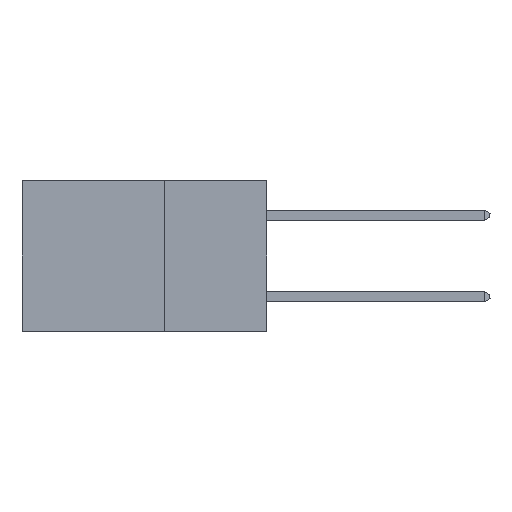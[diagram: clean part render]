
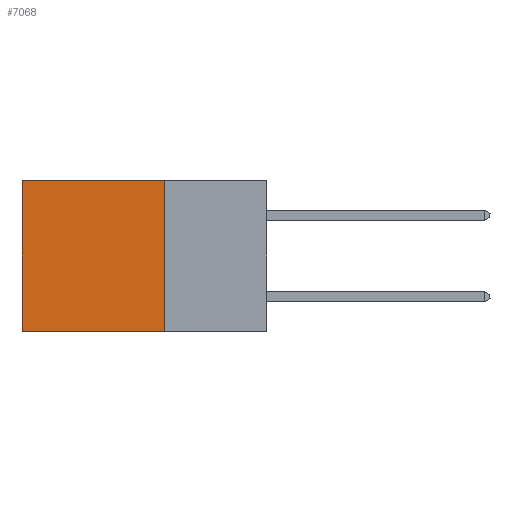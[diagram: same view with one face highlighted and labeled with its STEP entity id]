
A CAD part, left-side view. The second image highlights one B-rep face of the part: STEP entity #7068.
In plain terms, the highlighted planar face has unit normal (-1, 0, 0).
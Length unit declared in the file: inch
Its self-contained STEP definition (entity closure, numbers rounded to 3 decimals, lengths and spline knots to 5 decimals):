
#1151 = CARTESIAN_POINT ( 'NONE',  ( 0.2875, 0.25, 0. ) ) ;
#1280 = CARTESIAN_POINT ( 'NONE',  ( 0.2875, 0.25, -0.37 ) ) ;
#2963 = DIRECTION ( 'NONE',  ( 0., 0., -1. ) ) ;
#4629 = DIRECTION ( 'NONE',  ( 1., 0., 0. ) ) ;
#5916 = CARTESIAN_POINT ( 'NONE',  ( 0.2875, 0.25, 0. ) ) ;
#7068 = ADVANCED_FACE ( 'NONE', ( #40248 ), #21958, .F. ) ;
#8092 = EDGE_CURVE ( 'NONE', #14095, #40239, #42843, .T. ) ;
#14095 = VERTEX_POINT ( 'NONE', #38770 ) ;
#14405 = VERTEX_POINT ( 'NONE', #30082 ) ;
#14939 = ORIENTED_EDGE ( 'NONE', *, *, #38600, .T. ) ;
#16433 = DIRECTION ( 'NONE',  ( 0., 0., -1. ) ) ;
#17549 = LINE ( 'NONE', #37400, #34756 ) ;
#18613 = DIRECTION ( 'NONE',  ( 0., 1., 0. ) ) ;
#20931 = EDGE_CURVE ( 'NONE', #40239, #34434, #23187, .T. ) ;
#21083 = CARTESIAN_POINT ( 'NONE',  ( 0.2875, 0.6, -0.37 ) ) ;
#21958 = PLANE ( 'NONE',  #38261 ) ;
#23187 = LINE ( 'NONE', #1280, #41395 ) ;
#25270 = VECTOR ( 'NONE', #30795, 39.37008 ) ;
#27459 = EDGE_LOOP ( 'NONE', ( #14939, #30585, #40939, #38949 ) ) ;
#28905 = DIRECTION ( 'NONE',  ( 0., 0., -1. ) ) ;
#30082 = CARTESIAN_POINT ( 'NONE',  ( 0.2875, 0.6, 0. ) ) ;
#30585 = ORIENTED_EDGE ( 'NONE', *, *, #20931, .F. ) ;
#30795 = DIRECTION ( 'NONE',  ( 0., 1., 0. ) ) ;
#32689 = VECTOR ( 'NONE', #16433, 39.37008 ) ;
#32819 = CARTESIAN_POINT ( 'NONE',  ( 0.2875, 0.25, -0.37 ) ) ;
#34368 = LINE ( 'NONE', #40932, #25270 ) ;
#34434 = VERTEX_POINT ( 'NONE', #21083 ) ;
#34756 = VECTOR ( 'NONE', #2963, 39.37008 ) ;
#37015 = EDGE_CURVE ( 'NONE', #14095, #14405, #34368, .T. ) ;
#37400 = CARTESIAN_POINT ( 'NONE',  ( 0.2875, 0.6, 0. ) ) ;
#38261 = AXIS2_PLACEMENT_3D ( 'NONE', #1151, #4629, #28905 ) ;
#38600 = EDGE_CURVE ( 'NONE', #14405, #34434, #17549, .T. ) ;
#38770 = CARTESIAN_POINT ( 'NONE',  ( 0.2875, 0.25, 0. ) ) ;
#38949 = ORIENTED_EDGE ( 'NONE', *, *, #37015, .T. ) ;
#40239 = VERTEX_POINT ( 'NONE', #32819 ) ;
#40248 = FACE_OUTER_BOUND ( 'NONE', #27459, .T. ) ;
#40932 = CARTESIAN_POINT ( 'NONE',  ( 0.2875, 0.25, 0. ) ) ;
#40939 = ORIENTED_EDGE ( 'NONE', *, *, #8092, .F. ) ;
#41395 = VECTOR ( 'NONE', #18613, 39.37008 ) ;
#42843 = LINE ( 'NONE', #5916, #32689 ) ;
